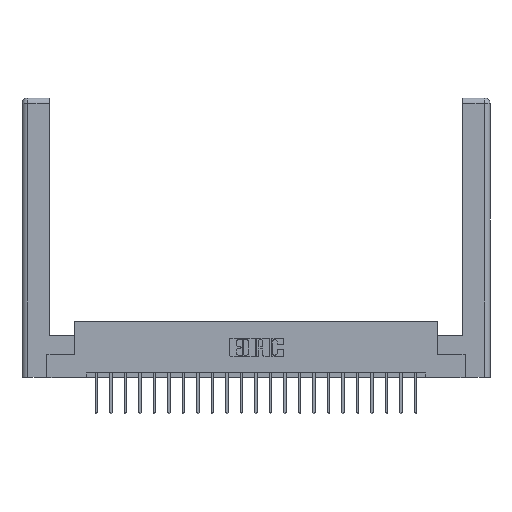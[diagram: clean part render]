
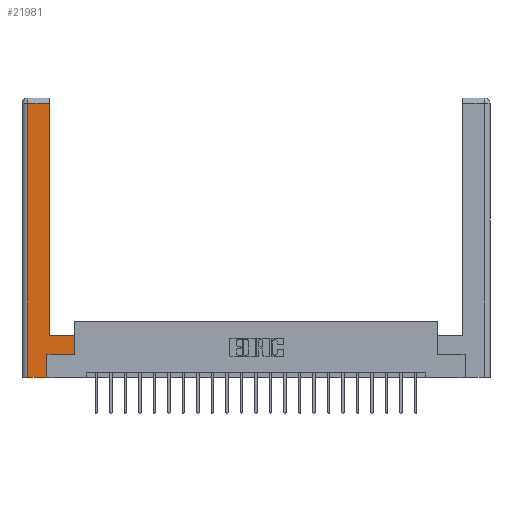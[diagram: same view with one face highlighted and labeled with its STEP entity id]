
A CAD part, top view. The second image highlights one B-rep face of the part: STEP entity #21981.
In plain terms, the highlighted planar face has unit normal (0, 0, 1).
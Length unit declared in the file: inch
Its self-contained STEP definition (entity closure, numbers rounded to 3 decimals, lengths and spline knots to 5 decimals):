
#177 = AXIS2_PLACEMENT_3D ( 'NONE', #11796, #1224, #6524 ) ;
#540 = DIRECTION ( 'NONE',  ( 0., 1., 0. ) ) ;
#1057 = VECTOR ( 'NONE', #2343, 39.37008 ) ;
#1224 = DIRECTION ( 'NONE',  ( 0., 0., -1. ) ) ;
#1756 = CARTESIAN_POINT ( 'NONE',  ( 0.565, 0.45, 0. ) ) ;
#1827 = LINE ( 'NONE', #1756, #13689 ) ;
#1836 = CARTESIAN_POINT ( 'NONE',  ( 0.565, 0.245, 0. ) ) ;
#1962 = VECTOR ( 'NONE', #15356, 39.37008 ) ;
#2089 = CARTESIAN_POINT ( 'NONE',  ( 0.265, 0.245, 0. ) ) ;
#2343 = DIRECTION ( 'NONE',  ( 1., 0., 0. ) ) ;
#2533 = VECTOR ( 'NONE', #16823, 39.37008 ) ;
#3221 = CARTESIAN_POINT ( 'NONE',  ( 0.565, 0.245, 0. ) ) ;
#3268 = EDGE_LOOP ( 'NONE', ( #16720, #8746, #11520, #21574, #20613, #6691, #20760, #8859 ) ) ;
#3707 = EDGE_CURVE ( 'NONE', #6443, #11782, #1827, .T. ) ;
#5027 = EDGE_CURVE ( 'NONE', #21448, #6443, #20899, .T. ) ;
#5037 = LINE ( 'NONE', #11767, #1962 ) ;
#6215 = EDGE_CURVE ( 'NONE', #21737, #21728, #11620, .T. ) ;
#6298 = EDGE_CURVE ( 'NONE', #21688, #10990, #5037, .T. ) ;
#6443 = VERTEX_POINT ( 'NONE', #3221 ) ;
#6524 = DIRECTION ( 'NONE',  ( -1., 0., 0. ) ) ;
#6691 = ORIENTED_EDGE ( 'NONE', *, *, #5027, .T. ) ;
#7301 = DIRECTION ( 'NONE',  ( -1., 0., 0. ) ) ;
#7610 = CARTESIAN_POINT ( 'NONE',  ( 0.0615, 0., 0. ) ) ;
#8601 = EDGE_CURVE ( 'NONE', #19444, #21448, #11342, .T. ) ;
#8746 = ORIENTED_EDGE ( 'NONE', *, *, #15408, .T. ) ;
#8859 = ORIENTED_EDGE ( 'NONE', *, *, #19264, .T. ) ;
#9829 = VECTOR ( 'NONE', #7301, 39.37008 ) ;
#10668 = EDGE_CURVE ( 'NONE', #21728, #19444, #11272, .T. ) ;
#10990 = VERTEX_POINT ( 'NONE', #13517 ) ;
#11272 = LINE ( 'NONE', #14406, #1057 ) ;
#11342 = LINE ( 'NONE', #2089, #17142 ) ;
#11520 = ORIENTED_EDGE ( 'NONE', *, *, #6215, .T. ) ;
#11620 = LINE ( 'NONE', #13426, #2533 ) ;
#11767 = CARTESIAN_POINT ( 'NONE',  ( 0.295, 3., 0. ) ) ;
#11782 = VERTEX_POINT ( 'NONE', #13331 ) ;
#11796 = CARTESIAN_POINT ( 'NONE',  ( 0., 0., 0. ) ) ;
#12840 = CARTESIAN_POINT ( 'NONE',  ( 0.295, 0.45, 0. ) ) ;
#13331 = CARTESIAN_POINT ( 'NONE',  ( 0.565, 0.45, 0. ) ) ;
#13426 = CARTESIAN_POINT ( 'NONE',  ( 0.0615, 0., 0. ) ) ;
#13517 = CARTESIAN_POINT ( 'NONE',  ( 0.295, 2.94, 0. ) ) ;
#13689 = VECTOR ( 'NONE', #19419, 39.37008 ) ;
#14197 = DIRECTION ( 'NONE',  ( 1., 0., 0. ) ) ;
#14406 = CARTESIAN_POINT ( 'NONE',  ( 0.265, 0., 0. ) ) ;
#15356 = DIRECTION ( 'NONE',  ( 0., 1., 0. ) ) ;
#15408 = EDGE_CURVE ( 'NONE', #10990, #21737, #18893, .T. ) ;
#15560 = CARTESIAN_POINT ( 'NONE',  ( 0.265, 0.245, 0. ) ) ;
#16047 = DIRECTION ( 'NONE',  ( -1., 0., 0. ) ) ;
#16720 = ORIENTED_EDGE ( 'NONE', *, *, #6298, .T. ) ;
#16823 = DIRECTION ( 'NONE',  ( 0., -1., 0. ) ) ;
#17140 = CARTESIAN_POINT ( 'NONE',  ( 0.0615, 2.94, 0. ) ) ;
#17142 = VECTOR ( 'NONE', #540, 39.37008 ) ;
#17172 = FACE_OUTER_BOUND ( 'NONE', #3268, .T. ) ;
#17500 = VECTOR ( 'NONE', #14197, 39.37008 ) ;
#18309 = VECTOR ( 'NONE', #16047, 39.37008 ) ;
#18713 = LINE ( 'NONE', #21493, #9829 ) ;
#18887 = CARTESIAN_POINT ( 'NONE',  ( 0.265, 0., 0. ) ) ;
#18893 = LINE ( 'NONE', #17140, #18309 ) ;
#18966 = PLANE ( 'NONE',  #177 ) ;
#19264 = EDGE_CURVE ( 'NONE', #11782, #21688, #18713, .T. ) ;
#19419 = DIRECTION ( 'NONE',  ( 0., 1., 0. ) ) ;
#19444 = VERTEX_POINT ( 'NONE', #18887 ) ;
#19783 = CARTESIAN_POINT ( 'NONE',  ( 0.0615, 2.94, 0. ) ) ;
#20613 = ORIENTED_EDGE ( 'NONE', *, *, #8601, .T. ) ;
#20760 = ORIENTED_EDGE ( 'NONE', *, *, #3707, .T. ) ;
#20899 = LINE ( 'NONE', #1836, #17500 ) ;
#21448 = VERTEX_POINT ( 'NONE', #15560 ) ;
#21493 = CARTESIAN_POINT ( 'NONE',  ( 0.295, 0.45, 0. ) ) ;
#21574 = ORIENTED_EDGE ( 'NONE', *, *, #10668, .T. ) ;
#21688 = VERTEX_POINT ( 'NONE', #12840 ) ;
#21728 = VERTEX_POINT ( 'NONE', #7610 ) ;
#21737 = VERTEX_POINT ( 'NONE', #19783 ) ;
#21981 = ADVANCED_FACE ( 'NONE', ( #17172 ), #18966, .F. ) ;
